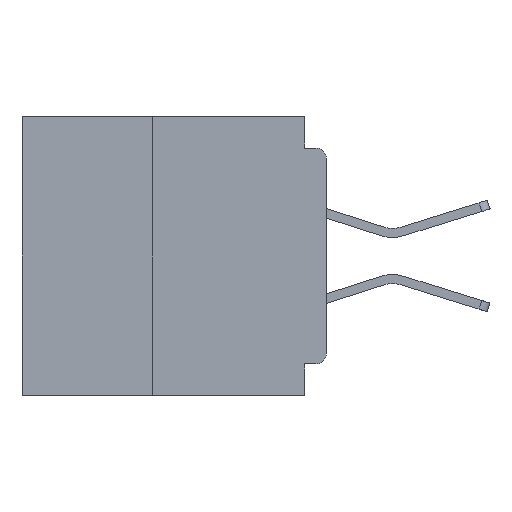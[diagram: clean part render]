
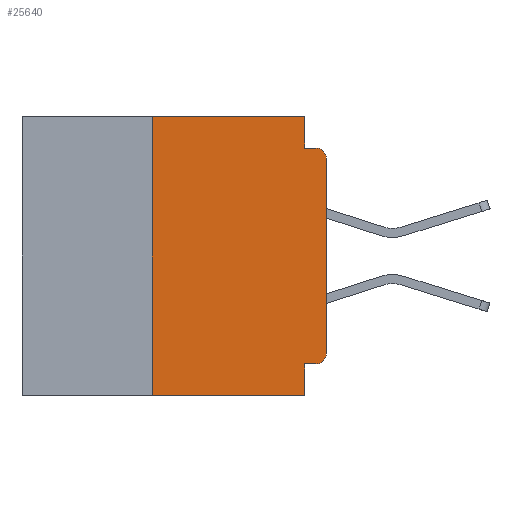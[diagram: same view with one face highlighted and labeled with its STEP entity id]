
A CAD part, left-side view. The second image highlights one B-rep face of the part: STEP entity #25640.
In plain terms, the highlighted planar face has unit normal (-1, 0, 0).
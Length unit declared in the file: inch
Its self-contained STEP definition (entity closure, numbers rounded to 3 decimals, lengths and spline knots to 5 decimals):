
#535 = ORIENTED_EDGE ( 'NONE', *, *, #30879, .F. ) ;
#1536 = CIRCLE ( 'NONE', #17524, 0.015 ) ;
#1922 = DIRECTION ( 'NONE',  ( 0., -1., 0. ) ) ;
#3595 = CARTESIAN_POINT ( 'NONE',  ( 0., 0.015, -0.045 ) ) ;
#3635 = LINE ( 'NONE', #33452, #29722 ) ;
#4010 = EDGE_LOOP ( 'NONE', ( #4873, #19077, #4208, #26651, #9963, #6496, #39472, #535, #15969, #10219 ) ) ;
#4208 = ORIENTED_EDGE ( 'NONE', *, *, #42512, .F. ) ;
#4873 = ORIENTED_EDGE ( 'NONE', *, *, #32713, .T. ) ;
#6085 = VECTOR ( 'NONE', #33180, 39.37008 ) ;
#6208 = EDGE_CURVE ( 'NONE', #14313, #19974, #27260, .T. ) ;
#6496 = ORIENTED_EDGE ( 'NONE', *, *, #20534, .F. ) ;
#7229 = EDGE_CURVE ( 'NONE', #26375, #37866, #1536, .T. ) ;
#7675 = CARTESIAN_POINT ( 'NONE',  ( 0., 0.031, 0. ) ) ;
#7825 = DIRECTION ( 'NONE',  ( -1., 0., 0. ) ) ;
#8244 = LINE ( 'NONE', #31292, #17364 ) ;
#8967 = CARTESIAN_POINT ( 'NONE',  ( 0., 0.031, -0.355 ) ) ;
#9721 = DIRECTION ( 'NONE',  ( 0., 0., -1. ) ) ;
#9872 = EDGE_CURVE ( 'NONE', #31034, #32948, #3635, .T. ) ;
#9963 = ORIENTED_EDGE ( 'NONE', *, *, #31203, .F. ) ;
#10219 = ORIENTED_EDGE ( 'NONE', *, *, #6208, .T. ) ;
#10548 = CARTESIAN_POINT ( 'NONE',  ( 0., 0.031, -0.4 ) ) ;
#11670 = VERTEX_POINT ( 'NONE', #8967 ) ;
#14313 = VERTEX_POINT ( 'NONE', #35055 ) ;
#14463 = PLANE ( 'NONE',  #38392 ) ;
#15072 = CARTESIAN_POINT ( 'NONE',  ( 0., 0.25, 0. ) ) ;
#15164 = LINE ( 'NONE', #19608, #6085 ) ;
#15697 = VERTEX_POINT ( 'NONE', #15072 ) ;
#15969 = ORIENTED_EDGE ( 'NONE', *, *, #42148, .F. ) ;
#15987 = VECTOR ( 'NONE', #24266, 39.37008 ) ;
#17067 = LINE ( 'NONE', #30902, #15987 ) ;
#17364 = VECTOR ( 'NONE', #37836, 39.37008 ) ;
#17524 = AXIS2_PLACEMENT_3D ( 'NONE', #28184, #7825, #31585 ) ;
#18341 = LINE ( 'NONE', #22406, #35221 ) ;
#18666 = DIRECTION ( 'NONE',  ( -1., 0., 0. ) ) ;
#18742 = CARTESIAN_POINT ( 'NONE',  ( 0., 0.437, -0.4 ) ) ;
#19040 = LINE ( 'NONE', #10548, #28034 ) ;
#19077 = ORIENTED_EDGE ( 'NONE', *, *, #7229, .T. ) ;
#19608 = CARTESIAN_POINT ( 'NONE',  ( 0., 0., -0.355 ) ) ;
#19974 = VERTEX_POINT ( 'NONE', #28646 ) ;
#20534 = EDGE_CURVE ( 'NONE', #21622, #15697, #17067, .T. ) ;
#21332 = DIRECTION ( 'NONE',  ( 0., 0., -1. ) ) ;
#21622 = VERTEX_POINT ( 'NONE', #29772 ) ;
#22406 = CARTESIAN_POINT ( 'NONE',  ( 0., 0., -0.045 ) ) ;
#24046 = CARTESIAN_POINT ( 'NONE',  ( 0., 0.031, -0.4 ) ) ;
#24091 = FACE_OUTER_BOUND ( 'NONE', #4010, .T. ) ;
#24266 = DIRECTION ( 'NONE',  ( 0., 0., 1. ) ) ;
#25640 = ADVANCED_FACE ( 'NONE', ( #24091 ), #14463, .F. ) ;
#26375 = VERTEX_POINT ( 'NONE', #27669 ) ;
#26651 = ORIENTED_EDGE ( 'NONE', *, *, #9872, .F. ) ;
#27141 = EDGE_CURVE ( 'NONE', #21622, #29698, #43278, .T. ) ;
#27260 = CIRCLE ( 'NONE', #43341, 0.015 ) ;
#27482 = DIRECTION ( 'NONE',  ( 0., 0., -1. ) ) ;
#27669 = CARTESIAN_POINT ( 'NONE',  ( 0., 0., -0.06 ) ) ;
#28034 = VECTOR ( 'NONE', #27482, 39.37008 ) ;
#28184 = CARTESIAN_POINT ( 'NONE',  ( 0., 0.015, -0.06 ) ) ;
#28646 = CARTESIAN_POINT ( 'NONE',  ( 0., 0., -0.34 ) ) ;
#29698 = VERTEX_POINT ( 'NONE', #24046 ) ;
#29722 = VECTOR ( 'NONE', #9721, 39.37008 ) ;
#29772 = CARTESIAN_POINT ( 'NONE',  ( 0., 0.25, -0.4 ) ) ;
#30879 = EDGE_CURVE ( 'NONE', #11670, #29698, #19040, .T. ) ;
#30902 = CARTESIAN_POINT ( 'NONE',  ( 0., 0.25, -0.4 ) ) ;
#31034 = VERTEX_POINT ( 'NONE', #7675 ) ;
#31203 = EDGE_CURVE ( 'NONE', #15697, #31034, #34340, .T. ) ;
#31292 = CARTESIAN_POINT ( 'NONE',  ( 0., 0., 0. ) ) ;
#31585 = DIRECTION ( 'NONE',  ( 0., 0., -1. ) ) ;
#32315 = CARTESIAN_POINT ( 'NONE',  ( 0., 0.437, 0. ) ) ;
#32713 = EDGE_CURVE ( 'NONE', #19974, #26375, #8244, .T. ) ;
#32948 = VERTEX_POINT ( 'NONE', #35798 ) ;
#33180 = DIRECTION ( 'NONE',  ( 0., 1., 0. ) ) ;
#33452 = CARTESIAN_POINT ( 'NONE',  ( 0., 0.031, 0. ) ) ;
#34340 = LINE ( 'NONE', #32315, #36415 ) ;
#34478 = VECTOR ( 'NONE', #38878, 39.37008 ) ;
#35055 = CARTESIAN_POINT ( 'NONE',  ( 0., 0.015, -0.355 ) ) ;
#35221 = VECTOR ( 'NONE', #1922, 39.37008 ) ;
#35798 = CARTESIAN_POINT ( 'NONE',  ( 0., 0.031, -0.045 ) ) ;
#36415 = VECTOR ( 'NONE', #42342, 39.37008 ) ;
#37836 = DIRECTION ( 'NONE',  ( 0., 0., 1. ) ) ;
#37866 = VERTEX_POINT ( 'NONE', #3595 ) ;
#38050 = CARTESIAN_POINT ( 'NONE',  ( 0., 0.437, 0. ) ) ;
#38392 = AXIS2_PLACEMENT_3D ( 'NONE', #38050, #41411, #21332 ) ;
#38797 = CARTESIAN_POINT ( 'NONE',  ( 0., 0.015, -0.34 ) ) ;
#38878 = DIRECTION ( 'NONE',  ( 0., -1., 0. ) ) ;
#39472 = ORIENTED_EDGE ( 'NONE', *, *, #27141, .T. ) ;
#41411 = DIRECTION ( 'NONE',  ( 1., 0., 0. ) ) ;
#42136 = DIRECTION ( 'NONE',  ( 0., 0., -1. ) ) ;
#42148 = EDGE_CURVE ( 'NONE', #14313, #11670, #15164, .T. ) ;
#42342 = DIRECTION ( 'NONE',  ( 0., -1., 0. ) ) ;
#42512 = EDGE_CURVE ( 'NONE', #32948, #37866, #18341, .T. ) ;
#43278 = LINE ( 'NONE', #18742, #34478 ) ;
#43341 = AXIS2_PLACEMENT_3D ( 'NONE', #38797, #18666, #42136 ) ;
